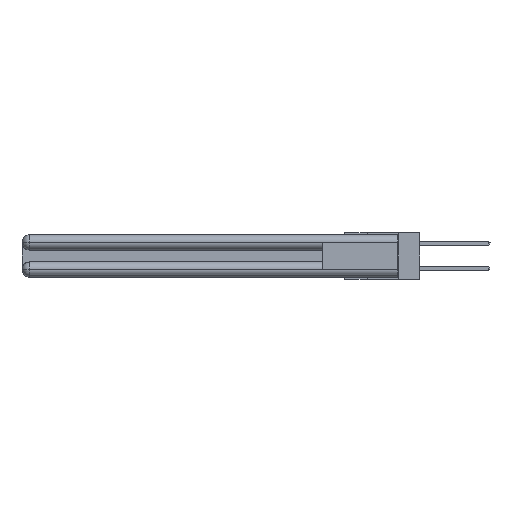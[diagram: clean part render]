
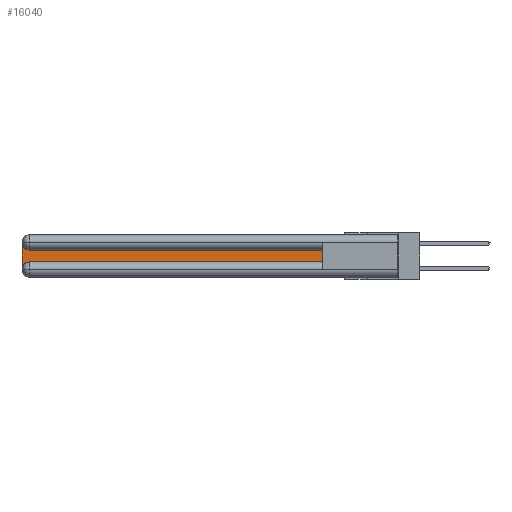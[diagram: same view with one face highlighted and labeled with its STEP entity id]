
A CAD part, left-side view. The second image highlights one B-rep face of the part: STEP entity #16040.
In plain terms, the highlighted planar face has unit normal (-1, 0, 0).
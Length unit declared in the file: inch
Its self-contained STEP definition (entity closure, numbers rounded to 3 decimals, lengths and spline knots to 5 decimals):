
#51 = CARTESIAN_POINT ( 'NONE',  ( 0.075, 0.6, -0.1225 ) ) ;
#329 = CARTESIAN_POINT ( 'NONE',  ( 0.075, 3., -0.0625 ) ) ;
#1439 = VECTOR ( 'NONE', #25212, 39.37008 ) ;
#1823 = CARTESIAN_POINT ( 'NONE',  ( 0.075, 3., -0.1225 ) ) ;
#2029 = AXIS2_PLACEMENT_3D ( 'NONE', #2096, #26898, #31489 ) ;
#2065 = ORIENTED_EDGE ( 'NONE', *, *, #17189, .T. ) ;
#2096 = CARTESIAN_POINT ( 'NONE',  ( 0.075, 2.94, -0.2775 ) ) ;
#3184 = VERTEX_POINT ( 'NONE', #16678 ) ;
#3595 = EDGE_CURVE ( 'NONE', #31005, #3184, #12881, .T. ) ;
#3963 = VERTEX_POINT ( 'NONE', #8812 ) ;
#4132 = DIRECTION ( 'NONE',  ( 1., 0., 0. ) ) ;
#4717 = CARTESIAN_POINT ( 'NONE',  ( 0.075, 2.94, -0.0625 ) ) ;
#5077 = DIRECTION ( 'NONE',  ( 0., 1., 0. ) ) ;
#6002 = ORIENTED_EDGE ( 'NONE', *, *, #13554, .T. ) ;
#7676 = EDGE_CURVE ( 'NONE', #3184, #22148, #21901, .T. ) ;
#8812 = CARTESIAN_POINT ( 'NONE',  ( 0.075, 0.6, -0.1225 ) ) ;
#9029 = PLANE ( 'NONE',  #28839 ) ;
#9110 = EDGE_LOOP ( 'NONE', ( #6002, #21041, #2065, #19741, #23725, #28356 ) ) ;
#9398 = DIRECTION ( 'NONE',  ( 0., 0., -1. ) ) ;
#9668 = DIRECTION ( 'NONE',  ( 0., -1., 0. ) ) ;
#11196 = VECTOR ( 'NONE', #5077, 39.37008 ) ;
#11259 = CARTESIAN_POINT ( 'NONE',  ( 0.075, 0.6, -0.2175 ) ) ;
#12772 = FACE_OUTER_BOUND ( 'NONE', #9110, .T. ) ;
#12881 = CIRCLE ( 'NONE', #2029, 0.06 ) ;
#13554 = EDGE_CURVE ( 'NONE', #3963, #30699, #13916, .T. ) ;
#13916 = LINE ( 'NONE', #51, #11196 ) ;
#15788 = VECTOR ( 'NONE', #15831, 39.37008 ) ;
#15831 = DIRECTION ( 'NONE',  ( 0., 0., -1. ) ) ;
#16040 = ADVANCED_FACE ( 'NONE', ( #12772 ), #9029, .F. ) ;
#16148 = LINE ( 'NONE', #30700, #15788 ) ;
#16678 = CARTESIAN_POINT ( 'NONE',  ( 0.075, 2.94, -0.2175 ) ) ;
#17131 = DIRECTION ( 'NONE',  ( 1., 0., 0. ) ) ;
#17189 = EDGE_CURVE ( 'NONE', #31049, #31005, #16148, .T. ) ;
#17272 = CARTESIAN_POINT ( 'NONE',  ( 0.075, 2.94, -0.1225 ) ) ;
#17435 = EDGE_CURVE ( 'NONE', #22148, #3963, #23139, .T. ) ;
#18818 = VECTOR ( 'NONE', #9668, 39.37008 ) ;
#18952 = DIRECTION ( 'NONE',  ( 0., 0., -1. ) ) ;
#19741 = ORIENTED_EDGE ( 'NONE', *, *, #3595, .T. ) ;
#20150 = CARTESIAN_POINT ( 'NONE',  ( 0.075, 3., -0.2775 ) ) ;
#20303 = CIRCLE ( 'NONE', #22864, 0.06 ) ;
#21041 = ORIENTED_EDGE ( 'NONE', *, *, #26959, .T. ) ;
#21527 = CARTESIAN_POINT ( 'NONE',  ( 0.075, 0.6, -0.2175 ) ) ;
#21901 = LINE ( 'NONE', #21527, #18818 ) ;
#22148 = VERTEX_POINT ( 'NONE', #11259 ) ;
#22864 = AXIS2_PLACEMENT_3D ( 'NONE', #4717, #17131, #9398 ) ;
#23139 = LINE ( 'NONE', #24344, #1439 ) ;
#23725 = ORIENTED_EDGE ( 'NONE', *, *, #7676, .T. ) ;
#24344 = CARTESIAN_POINT ( 'NONE',  ( 0.075, 0.6, -0.2175 ) ) ;
#25212 = DIRECTION ( 'NONE',  ( 0., 0., 1. ) ) ;
#26898 = DIRECTION ( 'NONE',  ( 1., 0., 0. ) ) ;
#26959 = EDGE_CURVE ( 'NONE', #30699, #31049, #20303, .T. ) ;
#28356 = ORIENTED_EDGE ( 'NONE', *, *, #17435, .T. ) ;
#28839 = AXIS2_PLACEMENT_3D ( 'NONE', #1823, #4132, #18952 ) ;
#30699 = VERTEX_POINT ( 'NONE', #17272 ) ;
#30700 = CARTESIAN_POINT ( 'NONE',  ( 0.075, 3., -0.2175 ) ) ;
#31005 = VERTEX_POINT ( 'NONE', #20150 ) ;
#31049 = VERTEX_POINT ( 'NONE', #329 ) ;
#31489 = DIRECTION ( 'NONE',  ( 0., 0., -1. ) ) ;
